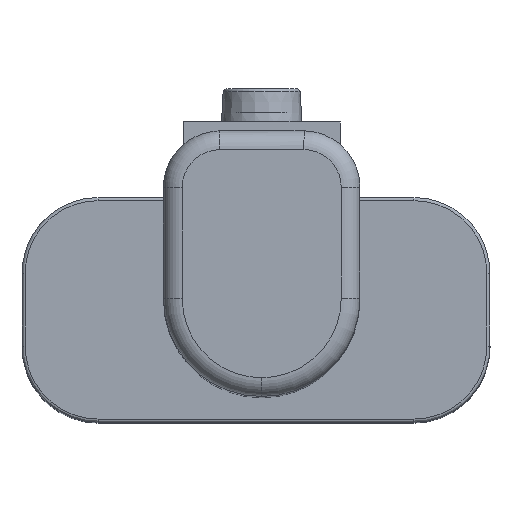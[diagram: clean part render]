
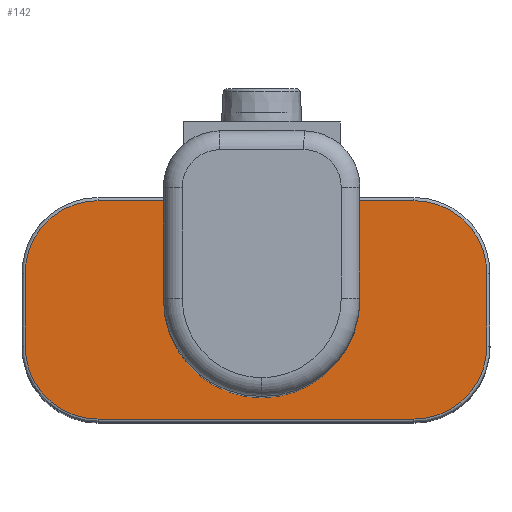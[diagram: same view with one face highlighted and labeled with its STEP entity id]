
A CAD part, top view. The second image highlights one B-rep face of the part: STEP entity #142.
In plain terms, the highlighted planar face has unit normal (0, 0, 1).
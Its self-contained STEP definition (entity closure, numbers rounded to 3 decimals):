
#41 = ORIENTED_EDGE ( 'NONE', *, *, #7471, .T. ) ;
#142 = ADVANCED_FACE ( 'NONE', ( #8301 ), #3641, .T. ) ;
#216 = EDGE_CURVE ( 'NONE', #11446, #6212, #11033, .T. ) ;
#373 = CIRCLE ( 'NONE', #2927, 2.336 ) ;
#378 = ORIENTED_EDGE ( 'NONE', *, *, #2096, .T. ) ;
#458 = VERTEX_POINT ( 'NONE', #9082 ) ;
#623 = VERTEX_POINT ( 'NONE', #7263 ) ;
#641 = LINE ( 'NONE', #8522, #8597 ) ;
#1117 = EDGE_CURVE ( 'NONE', #8200, #458, #7514, .T. ) ;
#1312 = DIRECTION ( 'NONE',  ( 0., 1., 0. ) ) ;
#1698 = CIRCLE ( 'NONE', #8073, 2.336 ) ;
#2096 = EDGE_CURVE ( 'NONE', #623, #11510, #5457, .T. ) ;
#2324 = VECTOR ( 'NONE', #1312, 1000. ) ;
#2547 = CARTESIAN_POINT ( 'NONE',  ( -5.247, 1.034, -124.385 ) ) ;
#2587 = DIRECTION ( 'NONE',  ( 0., 0., 1. ) ) ;
#2662 = DIRECTION ( 'NONE',  ( 0., -1., 0. ) ) ;
#2927 = AXIS2_PLACEMENT_3D ( 'NONE', #8386, #2587, #4448 ) ;
#3111 = CARTESIAN_POINT ( 'NONE',  ( 7.217, 1.034, -124.385 ) ) ;
#3322 = CIRCLE ( 'NONE', #4181, 2.336 ) ;
#3641 = PLANE ( 'NONE',  #11955 ) ;
#3691 = DIRECTION ( 'NONE',  ( 0., -1., 0. ) ) ;
#3793 = EDGE_CURVE ( 'NONE', #11510, #12554, #373, .T. ) ;
#3888 = LINE ( 'NONE', #10819, #10922 ) ;
#4181 = AXIS2_PLACEMENT_3D ( 'NONE', #6629, #10707, #3691 ) ;
#4448 = DIRECTION ( 'NONE',  ( 0., -1., 0. ) ) ;
#4943 = DIRECTION ( 'NONE',  ( 0., 0., 1. ) ) ;
#5147 = ORIENTED_EDGE ( 'NONE', *, *, #5464, .T. ) ;
#5444 = CARTESIAN_POINT ( 'NONE',  ( -5.247, 3.37, -124.385 ) ) ;
#5457 = LINE ( 'NONE', #11578, #2324 ) ;
#5464 = EDGE_CURVE ( 'NONE', #6212, #623, #1698, .T. ) ;
#5504 = ORIENTED_EDGE ( 'NONE', *, *, #11069, .T. ) ;
#5539 = ORIENTED_EDGE ( 'NONE', *, *, #3793, .T. ) ;
#5639 = CARTESIAN_POINT ( 'NONE',  ( 4.881, 3.37, -124.385 ) ) ;
#6212 = VERTEX_POINT ( 'NONE', #8259 ) ;
#6232 = VECTOR ( 'NONE', #12259, 1000. ) ;
#6539 = DIRECTION ( 'NONE',  ( 0., -1., 0. ) ) ;
#6629 = CARTESIAN_POINT ( 'NONE',  ( -5.247, -1.294, -124.385 ) ) ;
#6865 = AXIS2_PLACEMENT_3D ( 'NONE', #2547, #10620, #7449 ) ;
#6933 = CARTESIAN_POINT ( 'NONE',  ( 4.881, -1.294, -124.385 ) ) ;
#7263 = CARTESIAN_POINT ( 'NONE',  ( 7.217, -1.294, -124.385 ) ) ;
#7449 = DIRECTION ( 'NONE',  ( 0., -1., 0. ) ) ;
#7471 = EDGE_CURVE ( 'NONE', #7619, #11446, #3322, .T. ) ;
#7514 = CIRCLE ( 'NONE', #6865, 2.336 ) ;
#7619 = VERTEX_POINT ( 'NONE', #13238 ) ;
#7702 = DIRECTION ( 'NONE',  ( 0., 0., 1. ) ) ;
#8073 = AXIS2_PLACEMENT_3D ( 'NONE', #6933, #4943, #13089 ) ;
#8200 = VERTEX_POINT ( 'NONE', #5444 ) ;
#8259 = CARTESIAN_POINT ( 'NONE',  ( 4.881, -3.63, -124.385 ) ) ;
#8301 = FACE_OUTER_BOUND ( 'NONE', #11741, .T. ) ;
#8386 = CARTESIAN_POINT ( 'NONE',  ( 4.881, 1.034, -124.385 ) ) ;
#8522 = CARTESIAN_POINT ( 'NONE',  ( -7.583, -0.13, -124.385 ) ) ;
#8597 = VECTOR ( 'NONE', #6539, 1000. ) ;
#9082 = CARTESIAN_POINT ( 'NONE',  ( -7.583, 1.034, -124.385 ) ) ;
#9817 = DIRECTION ( 'NONE',  ( -1., 0., 0. ) ) ;
#10620 = DIRECTION ( 'NONE',  ( 0., 0., 1. ) ) ;
#10707 = DIRECTION ( 'NONE',  ( 0., 0., 1. ) ) ;
#10819 = CARTESIAN_POINT ( 'NONE',  ( -4.847, 3.37, -124.385 ) ) ;
#10847 = CARTESIAN_POINT ( 'NONE',  ( -7.583, -1.294, -124.385 ) ) ;
#10922 = VECTOR ( 'NONE', #9817, 1000. ) ;
#11033 = LINE ( 'NONE', #12110, #6232 ) ;
#11069 = EDGE_CURVE ( 'NONE', #12554, #8200, #3888, .T. ) ;
#11234 = CARTESIAN_POINT ( 'NONE',  ( -5.247, -3.63, -124.385 ) ) ;
#11385 = EDGE_CURVE ( 'NONE', #458, #7619, #641, .T. ) ;
#11446 = VERTEX_POINT ( 'NONE', #11234 ) ;
#11510 = VERTEX_POINT ( 'NONE', #3111 ) ;
#11578 = CARTESIAN_POINT ( 'NONE',  ( 7.217, 0.784, -124.385 ) ) ;
#11741 = EDGE_LOOP ( 'NONE', ( #11936, #41, #12902, #5147, #378, #5539, #5504, #12387 ) ) ;
#11936 = ORIENTED_EDGE ( 'NONE', *, *, #11385, .T. ) ;
#11955 = AXIS2_PLACEMENT_3D ( 'NONE', #10847, #7702, #2662 ) ;
#12110 = CARTESIAN_POINT ( 'NONE',  ( 4.881, -3.63, -124.385 ) ) ;
#12259 = DIRECTION ( 'NONE',  ( 1., 0., 0. ) ) ;
#12387 = ORIENTED_EDGE ( 'NONE', *, *, #1117, .T. ) ;
#12554 = VERTEX_POINT ( 'NONE', #5639 ) ;
#12902 = ORIENTED_EDGE ( 'NONE', *, *, #216, .T. ) ;
#13089 = DIRECTION ( 'NONE',  ( 0., -1., 0. ) ) ;
#13238 = CARTESIAN_POINT ( 'NONE',  ( -7.583, -1.294, -124.385 ) ) ;
